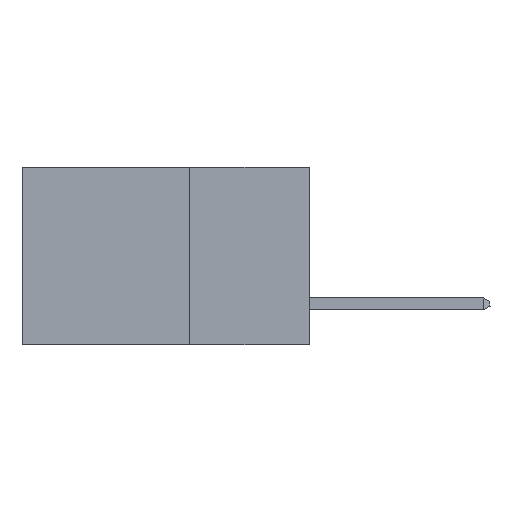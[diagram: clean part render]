
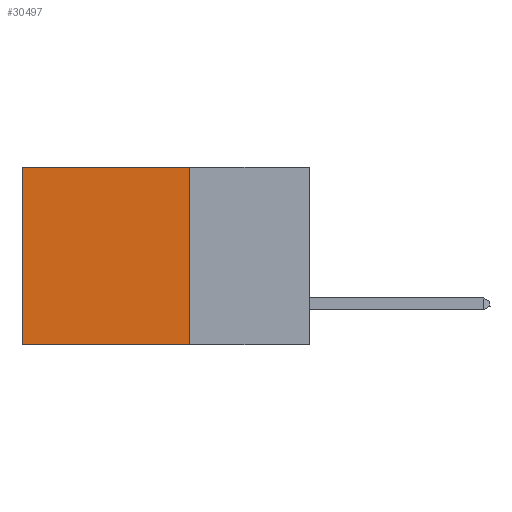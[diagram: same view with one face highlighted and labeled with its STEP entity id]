
A CAD part, left-side view. The second image highlights one B-rep face of the part: STEP entity #30497.
In plain terms, the highlighted planar face has unit normal (-1, 0, 0).
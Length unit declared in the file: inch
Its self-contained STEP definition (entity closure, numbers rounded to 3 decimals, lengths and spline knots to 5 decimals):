
#5161 = EDGE_CURVE ( 'NONE', #47386, #21135, #35236, .T. ) ;
#6729 = VERTEX_POINT ( 'NONE', #24040 ) ;
#7888 = FACE_OUTER_BOUND ( 'NONE', #39089, .T. ) ;
#9509 = PLANE ( 'NONE',  #32511 ) ;
#9814 = VECTOR ( 'NONE', #30185, 39.37008 ) ;
#10794 = CARTESIAN_POINT ( 'NONE',  ( 0.2875, 0.25, -0.37 ) ) ;
#13343 = LINE ( 'NONE', #46049, #9814 ) ;
#17481 = VECTOR ( 'NONE', #33520, 39.37008 ) ;
#19301 = ORIENTED_EDGE ( 'NONE', *, *, #43064, .F. ) ;
#21135 = VERTEX_POINT ( 'NONE', #37430 ) ;
#22207 = ORIENTED_EDGE ( 'NONE', *, *, #5161, .F. ) ;
#22446 = ORIENTED_EDGE ( 'NONE', *, *, #28886, .T. ) ;
#22659 = EDGE_CURVE ( 'NONE', #48653, #6729, #13343, .T. ) ;
#24040 = CARTESIAN_POINT ( 'NONE',  ( 0.2875, 0.6, 0. ) ) ;
#24217 = CARTESIAN_POINT ( 'NONE',  ( 0.2875, 0.25, 0. ) ) ;
#27542 = LINE ( 'NONE', #41574, #17481 ) ;
#28886 = EDGE_CURVE ( 'NONE', #6729, #21135, #27542, .T. ) ;
#29981 = CARTESIAN_POINT ( 'NONE',  ( 0.2875, 0.25, -0.37 ) ) ;
#30185 = DIRECTION ( 'NONE',  ( 0., 1., 0. ) ) ;
#30497 = ADVANCED_FACE ( 'NONE', ( #7888 ), #9509, .F. ) ;
#31468 = CARTESIAN_POINT ( 'NONE',  ( 0.2875, 0.25, 0. ) ) ;
#32511 = AXIS2_PLACEMENT_3D ( 'NONE', #24217, #43391, #46737 ) ;
#33520 = DIRECTION ( 'NONE',  ( 0., 0., -1. ) ) ;
#33705 = ORIENTED_EDGE ( 'NONE', *, *, #22659, .T. ) ;
#35236 = LINE ( 'NONE', #10794, #41116 ) ;
#37430 = CARTESIAN_POINT ( 'NONE',  ( 0.2875, 0.6, -0.37 ) ) ;
#39089 = EDGE_LOOP ( 'NONE', ( #22446, #22207, #19301, #33705 ) ) ;
#39209 = DIRECTION ( 'NONE',  ( 0., 0., -1. ) ) ;
#39719 = VECTOR ( 'NONE', #39209, 39.37008 ) ;
#41116 = VECTOR ( 'NONE', #45360, 39.37008 ) ;
#41574 = CARTESIAN_POINT ( 'NONE',  ( 0.2875, 0.6, 0. ) ) ;
#43064 = EDGE_CURVE ( 'NONE', #48653, #47386, #47419, .T. ) ;
#43391 = DIRECTION ( 'NONE',  ( 1., 0., 0. ) ) ;
#43829 = CARTESIAN_POINT ( 'NONE',  ( 0.2875, 0.25, 0. ) ) ;
#45360 = DIRECTION ( 'NONE',  ( 0., 1., 0. ) ) ;
#46049 = CARTESIAN_POINT ( 'NONE',  ( 0.2875, 0.25, 0. ) ) ;
#46737 = DIRECTION ( 'NONE',  ( 0., 0., -1. ) ) ;
#47386 = VERTEX_POINT ( 'NONE', #29981 ) ;
#47419 = LINE ( 'NONE', #31468, #39719 ) ;
#48653 = VERTEX_POINT ( 'NONE', #43829 ) ;
